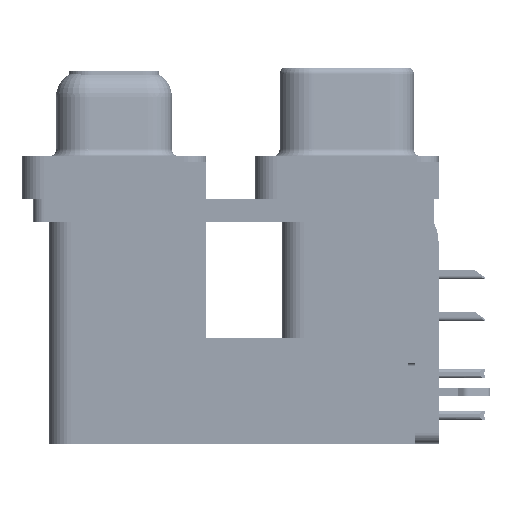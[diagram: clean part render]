
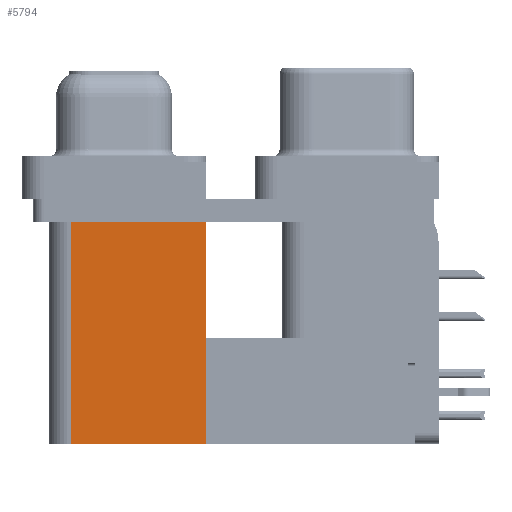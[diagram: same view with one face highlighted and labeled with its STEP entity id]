
A CAD part, left-side view. The second image highlights one B-rep face of the part: STEP entity #5794.
In plain terms, the highlighted planar face has unit normal (-1, 0, 0).
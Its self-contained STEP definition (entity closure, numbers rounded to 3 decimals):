
#3207 = VECTOR ( 'NONE', #56523, 1000. ) ;
#5440 = CARTESIAN_POINT ( 'NONE',  ( 3.7, 9.6, -19.2 ) ) ;
#5794 = ADVANCED_FACE ( 'NONE', ( #24061 ), #18724, .F. ) ;
#10996 = CARTESIAN_POINT ( 'NONE',  ( 3.7, 18.8, -19.2 ) ) ;
#12015 = LINE ( 'NONE', #33831, #3207 ) ;
#13440 = VECTOR ( 'NONE', #17368, 1000. ) ;
#16795 = CARTESIAN_POINT ( 'NONE',  ( 3.7, 9.6, -2.5 ) ) ;
#16923 = VERTEX_POINT ( 'NONE', #10996 ) ;
#17368 = DIRECTION ( 'NONE',  ( 0., 1., 0. ) ) ;
#18724 = PLANE ( 'NONE',  #20939 ) ;
#19290 = CARTESIAN_POINT ( 'NONE',  ( 3.7, 9.6, -19.2 ) ) ;
#19453 = ORIENTED_EDGE ( 'NONE', *, *, #20751, .F. ) ;
#20751 = EDGE_CURVE ( 'NONE', #16923, #22319, #35731, .T. ) ;
#20939 = AXIS2_PLACEMENT_3D ( 'NONE', #49442, #41585, #31910 ) ;
#22319 = VERTEX_POINT ( 'NONE', #51456 ) ;
#24061 = FACE_OUTER_BOUND ( 'NONE', #46904, .T. ) ;
#24597 = EDGE_CURVE ( 'NONE', #56563, #16923, #12015, .T. ) ;
#25974 = DIRECTION ( 'NONE',  ( 0., 0., 1. ) ) ;
#27575 = EDGE_CURVE ( 'NONE', #34529, #22319, #56128, .T. ) ;
#31596 = ORIENTED_EDGE ( 'NONE', *, *, #48715, .T. ) ;
#31910 = DIRECTION ( 'NONE',  ( 0., 0., -1. ) ) ;
#32466 = DIRECTION ( 'NONE',  ( 0., 0., 1. ) ) ;
#33831 = CARTESIAN_POINT ( 'NONE',  ( 3.7, 9.6, -19.2 ) ) ;
#34138 = ORIENTED_EDGE ( 'NONE', *, *, #24597, .F. ) ;
#34529 = VERTEX_POINT ( 'NONE', #42527 ) ;
#35731 = LINE ( 'NONE', #39726, #50824 ) ;
#38940 = VECTOR ( 'NONE', #32466, 1000. ) ;
#39726 = CARTESIAN_POINT ( 'NONE',  ( 3.7, 18.8, -19.2 ) ) ;
#41278 = ORIENTED_EDGE ( 'NONE', *, *, #27575, .T. ) ;
#41585 = DIRECTION ( 'NONE',  ( 1., 0., 0. ) ) ;
#42527 = CARTESIAN_POINT ( 'NONE',  ( 3.7, 9.6, -2.5 ) ) ;
#45403 = LINE ( 'NONE', #19290, #38940 ) ;
#46904 = EDGE_LOOP ( 'NONE', ( #41278, #19453, #34138, #31596 ) ) ;
#48715 = EDGE_CURVE ( 'NONE', #56563, #34529, #45403, .T. ) ;
#49442 = CARTESIAN_POINT ( 'NONE',  ( 3.7, 9.6, -19.2 ) ) ;
#50824 = VECTOR ( 'NONE', #25974, 1000. ) ;
#51456 = CARTESIAN_POINT ( 'NONE',  ( 3.7, 18.8, -2.5 ) ) ;
#56128 = LINE ( 'NONE', #16795, #13440 ) ;
#56523 = DIRECTION ( 'NONE',  ( 0., 1., 0. ) ) ;
#56563 = VERTEX_POINT ( 'NONE', #5440 ) ;
